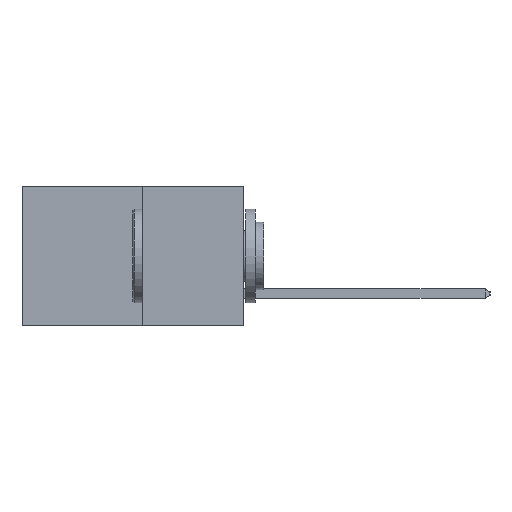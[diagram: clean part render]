
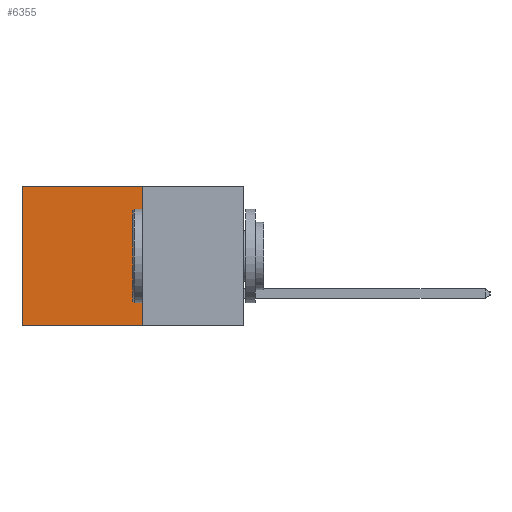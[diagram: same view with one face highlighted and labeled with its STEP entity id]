
A CAD part, left-side view. The second image highlights one B-rep face of the part: STEP entity #6355.
In plain terms, the highlighted planar face has unit normal (-1, 0, 0).
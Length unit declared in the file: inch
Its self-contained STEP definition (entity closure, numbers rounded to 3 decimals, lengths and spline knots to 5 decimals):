
#466 = ORIENTED_EDGE ( 'NONE', *, *, #4660, .T. ) ;
#871 = DIRECTION ( 'NONE',  ( 0., 1., 0. ) ) ;
#1237 = ORIENTED_EDGE ( 'NONE', *, *, #7318, .F. ) ;
#1514 = VECTOR ( 'NONE', #871, 39.37008 ) ;
#1710 = EDGE_LOOP ( 'NONE', ( #466, #1237, #2320, #5166 ) ) ;
#1835 = VECTOR ( 'NONE', #7901, 39.37008 ) ;
#2010 = LINE ( 'NONE', #4276, #10762 ) ;
#2320 = ORIENTED_EDGE ( 'NONE', *, *, #10779, .F. ) ;
#2798 = LINE ( 'NONE', #7252, #11230 ) ;
#2993 = CARTESIAN_POINT ( 'NONE',  ( 0.277, 0.27, 0. ) ) ;
#3420 = CARTESIAN_POINT ( 'NONE',  ( 0.277, 0.59, -0.37 ) ) ;
#3430 = DIRECTION ( 'NONE',  ( 1., 0., 0. ) ) ;
#3658 = CARTESIAN_POINT ( 'NONE',  ( 0.277, 0.27, -0.37 ) ) ;
#3830 = CARTESIAN_POINT ( 'NONE',  ( 0.277, 0.27, -0.37 ) ) ;
#3922 = LINE ( 'NONE', #9541, #1514 ) ;
#4276 = CARTESIAN_POINT ( 'NONE',  ( 0.277, 0.59, -0.37 ) ) ;
#4660 = EDGE_CURVE ( 'NONE', #6203, #6976, #2010, .T. ) ;
#5166 = ORIENTED_EDGE ( 'NONE', *, *, #10786, .T. ) ;
#5486 = VERTEX_POINT ( 'NONE', #3830 ) ;
#6203 = VERTEX_POINT ( 'NONE', #8357 ) ;
#6355 = ADVANCED_FACE ( 'NONE', ( #8453 ), #8543, .F. ) ;
#6638 = VERTEX_POINT ( 'NONE', #2993 ) ;
#6868 = CARTESIAN_POINT ( 'NONE',  ( 0.277, 0.27, -0.37 ) ) ;
#6976 = VERTEX_POINT ( 'NONE', #3420 ) ;
#7245 = DIRECTION ( 'NONE',  ( 0., 0., -1. ) ) ;
#7252 = CARTESIAN_POINT ( 'NONE',  ( 0.277, 0.27, -0.37 ) ) ;
#7318 = EDGE_CURVE ( 'NONE', #5486, #6976, #2798, .T. ) ;
#7319 = AXIS2_PLACEMENT_3D ( 'NONE', #6868, #3430, #9336 ) ;
#7901 = DIRECTION ( 'NONE',  ( 0., 0., -1. ) ) ;
#8357 = CARTESIAN_POINT ( 'NONE',  ( 0.277, 0.59, 0. ) ) ;
#8453 = FACE_OUTER_BOUND ( 'NONE', #1710, .T. ) ;
#8543 = PLANE ( 'NONE',  #7319 ) ;
#9336 = DIRECTION ( 'NONE',  ( 0., 0., -1. ) ) ;
#9541 = CARTESIAN_POINT ( 'NONE',  ( 0.277, 0.27, 0. ) ) ;
#10536 = DIRECTION ( 'NONE',  ( 0., 1., 0. ) ) ;
#10601 = LINE ( 'NONE', #3658, #1835 ) ;
#10762 = VECTOR ( 'NONE', #7245, 39.37008 ) ;
#10779 = EDGE_CURVE ( 'NONE', #6638, #5486, #10601, .T. ) ;
#10786 = EDGE_CURVE ( 'NONE', #6638, #6203, #3922, .T. ) ;
#11230 = VECTOR ( 'NONE', #10536, 39.37008 ) ;
